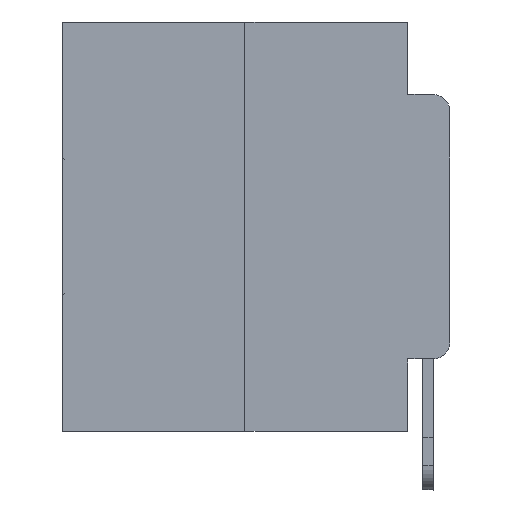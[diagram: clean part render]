
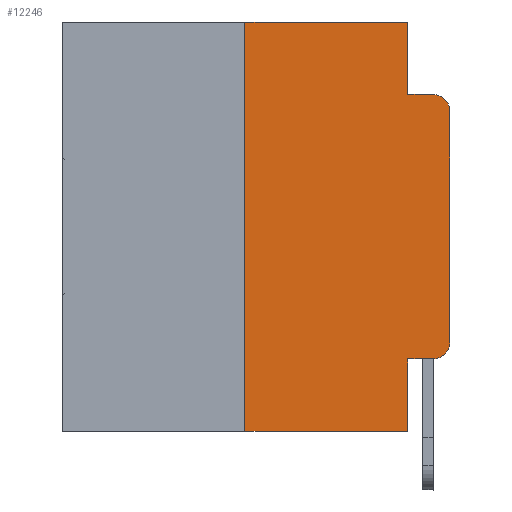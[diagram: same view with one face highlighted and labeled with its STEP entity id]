
A CAD part, left-side view. The second image highlights one B-rep face of the part: STEP entity #12246.
In plain terms, the highlighted planar face has unit normal (-1, 0, 0).
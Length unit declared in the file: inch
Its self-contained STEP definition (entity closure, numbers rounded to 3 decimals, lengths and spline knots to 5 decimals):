
#68 = DIRECTION ( 'NONE',  ( 0., -1., 0. ) ) ;
#430 = VECTOR ( 'NONE', #4182, 39.37008 ) ;
#444 = EDGE_CURVE ( 'NONE', #18312, #5038, #24142, .T. ) ;
#535 = ORIENTED_EDGE ( 'NONE', *, *, #27233, .F. ) ;
#691 = CARTESIAN_POINT ( 'NONE',  ( 0., 0.051, -0.0885 ) ) ;
#1001 = VERTEX_POINT ( 'NONE', #691 ) ;
#1068 = VECTOR ( 'NONE', #28125, 39.37008 ) ;
#2234 = DIRECTION ( 'NONE',  ( 0., 0., 1. ) ) ;
#2263 = EDGE_LOOP ( 'NONE', ( #26604, #11404, #8095, #535, #29459, #29853, #8856, #29320, #26165, #29931 ) ) ;
#2433 = CARTESIAN_POINT ( 'NONE',  ( 0., 0.473, -0.5 ) ) ;
#3103 = CARTESIAN_POINT ( 'NONE',  ( 0., 0.051, 0. ) ) ;
#3247 = DIRECTION ( 'NONE',  ( -1., 0., 0. ) ) ;
#3305 = DIRECTION ( 'NONE',  ( -1., 0., 0. ) ) ;
#3502 = AXIS2_PLACEMENT_3D ( 'NONE', #16220, #13831, #20787 ) ;
#3565 = CARTESIAN_POINT ( 'NONE',  ( 0., 0.051, 0. ) ) ;
#4182 = DIRECTION ( 'NONE',  ( 0., 0., 1. ) ) ;
#4618 = FACE_OUTER_BOUND ( 'NONE', #2263, .T. ) ;
#4714 = LINE ( 'NONE', #2433, #19577 ) ;
#5017 = EDGE_CURVE ( 'NONE', #7420, #17210, #7850, .T. ) ;
#5038 = VERTEX_POINT ( 'NONE', #3565 ) ;
#5615 = CARTESIAN_POINT ( 'NONE',  ( 0., 0.473, 0. ) ) ;
#6046 = CARTESIAN_POINT ( 'NONE',  ( 0., 0.051, 0. ) ) ;
#7420 = VERTEX_POINT ( 'NONE', #23541 ) ;
#7529 = EDGE_CURVE ( 'NONE', #18481, #22419, #4714, .T. ) ;
#7721 = AXIS2_PLACEMENT_3D ( 'NONE', #12750, #3305, #22320 ) ;
#7850 = LINE ( 'NONE', #18410, #430 ) ;
#7998 = VERTEX_POINT ( 'NONE', #20762 ) ;
#8095 = ORIENTED_EDGE ( 'NONE', *, *, #24989, .F. ) ;
#8517 = DIRECTION ( 'NONE',  ( 0., 0., -1. ) ) ;
#8735 = VECTOR ( 'NONE', #17221, 39.37008 ) ;
#8750 = VERTEX_POINT ( 'NONE', #9896 ) ;
#8856 = ORIENTED_EDGE ( 'NONE', *, *, #7529, .T. ) ;
#9086 = CARTESIAN_POINT ( 'NONE',  ( 0., 0.25, 0. ) ) ;
#9896 = CARTESIAN_POINT ( 'NONE',  ( 0., 0.02, -0.4115 ) ) ;
#10763 = CIRCLE ( 'NONE', #7721, 0.02 ) ;
#11080 = VECTOR ( 'NONE', #8517, 39.37008 ) ;
#11176 = VERTEX_POINT ( 'NONE', #19278 ) ;
#11404 = ORIENTED_EDGE ( 'NONE', *, *, #30465, .T. ) ;
#11756 = CARTESIAN_POINT ( 'NONE',  ( 0., 0.051, -0.4115 ) ) ;
#12076 = VECTOR ( 'NONE', #2234, 39.37008 ) ;
#12160 = CARTESIAN_POINT ( 'NONE',  ( 0., 0.25, -0.5 ) ) ;
#12246 = ADVANCED_FACE ( 'NONE', ( #4618 ), #30475, .F. ) ;
#12750 = CARTESIAN_POINT ( 'NONE',  ( 0., 0.02, -0.1085 ) ) ;
#13831 = DIRECTION ( 'NONE',  ( 1., 0., 0. ) ) ;
#14485 = DIRECTION ( 'NONE',  ( 0., -1., 0. ) ) ;
#14767 = DIRECTION ( 'NONE',  ( 0., -1., 0. ) ) ;
#15205 = LINE ( 'NONE', #11756, #1068 ) ;
#15353 = LINE ( 'NONE', #18982, #22792 ) ;
#16220 = CARTESIAN_POINT ( 'NONE',  ( 0., 0.473, 0. ) ) ;
#16748 = CARTESIAN_POINT ( 'NONE',  ( 0., 0.25, 0. ) ) ;
#17210 = VERTEX_POINT ( 'NONE', #21493 ) ;
#17221 = DIRECTION ( 'NONE',  ( 0., 0., -1. ) ) ;
#17678 = LINE ( 'NONE', #3103, #8735 ) ;
#18312 = VERTEX_POINT ( 'NONE', #16748 ) ;
#18410 = CARTESIAN_POINT ( 'NONE',  ( 0., 0., 0. ) ) ;
#18481 = VERTEX_POINT ( 'NONE', #12160 ) ;
#18982 = CARTESIAN_POINT ( 'NONE',  ( 0., 0.051, -0.0885 ) ) ;
#19278 = CARTESIAN_POINT ( 'NONE',  ( 0., 0.02, -0.0885 ) ) ;
#19577 = VECTOR ( 'NONE', #14485, 39.37008 ) ;
#19709 = EDGE_CURVE ( 'NONE', #7998, #22419, #17678, .T. ) ;
#19850 = DIRECTION ( 'NONE',  ( 0., 0., -1. ) ) ;
#20762 = CARTESIAN_POINT ( 'NONE',  ( 0., 0.051, -0.4115 ) ) ;
#20787 = DIRECTION ( 'NONE',  ( 0., 0., -1. ) ) ;
#21002 = LINE ( 'NONE', #9086, #12076 ) ;
#21049 = EDGE_CURVE ( 'NONE', #18481, #18312, #21002, .T. ) ;
#21493 = CARTESIAN_POINT ( 'NONE',  ( 0., 0., -0.1085 ) ) ;
#22320 = DIRECTION ( 'NONE',  ( 0., 0., -1. ) ) ;
#22419 = VERTEX_POINT ( 'NONE', #24131 ) ;
#22792 = VECTOR ( 'NONE', #68, 39.37008 ) ;
#23541 = CARTESIAN_POINT ( 'NONE',  ( 0., 0., -0.3915 ) ) ;
#24131 = CARTESIAN_POINT ( 'NONE',  ( 0., 0.051, -0.5 ) ) ;
#24142 = LINE ( 'NONE', #5615, #29735 ) ;
#24491 = LINE ( 'NONE', #6046, #11080 ) ;
#24989 = EDGE_CURVE ( 'NONE', #1001, #11176, #15353, .T. ) ;
#25826 = EDGE_CURVE ( 'NONE', #8750, #7420, #30548, .T. ) ;
#26165 = ORIENTED_EDGE ( 'NONE', *, *, #26786, .T. ) ;
#26290 = AXIS2_PLACEMENT_3D ( 'NONE', #26967, #3247, #19850 ) ;
#26604 = ORIENTED_EDGE ( 'NONE', *, *, #5017, .T. ) ;
#26786 = EDGE_CURVE ( 'NONE', #7998, #8750, #15205, .T. ) ;
#26967 = CARTESIAN_POINT ( 'NONE',  ( 0., 0.02, -0.3915 ) ) ;
#27233 = EDGE_CURVE ( 'NONE', #5038, #1001, #24491, .T. ) ;
#28125 = DIRECTION ( 'NONE',  ( 0., -1., 0. ) ) ;
#29320 = ORIENTED_EDGE ( 'NONE', *, *, #19709, .F. ) ;
#29459 = ORIENTED_EDGE ( 'NONE', *, *, #444, .F. ) ;
#29735 = VECTOR ( 'NONE', #14767, 39.37008 ) ;
#29853 = ORIENTED_EDGE ( 'NONE', *, *, #21049, .F. ) ;
#29931 = ORIENTED_EDGE ( 'NONE', *, *, #25826, .T. ) ;
#30465 = EDGE_CURVE ( 'NONE', #17210, #11176, #10763, .T. ) ;
#30475 = PLANE ( 'NONE',  #3502 ) ;
#30548 = CIRCLE ( 'NONE', #26290, 0.02 ) ;
